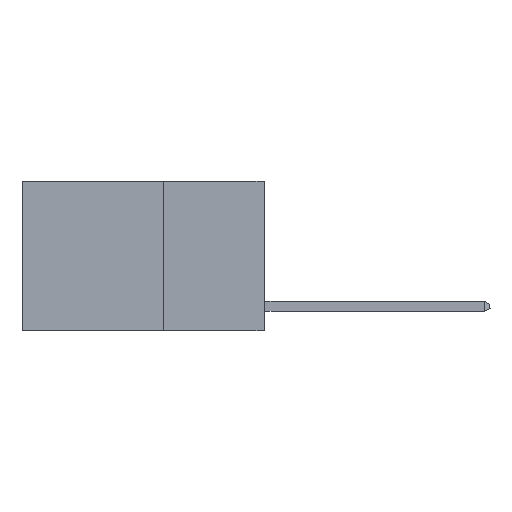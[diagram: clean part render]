
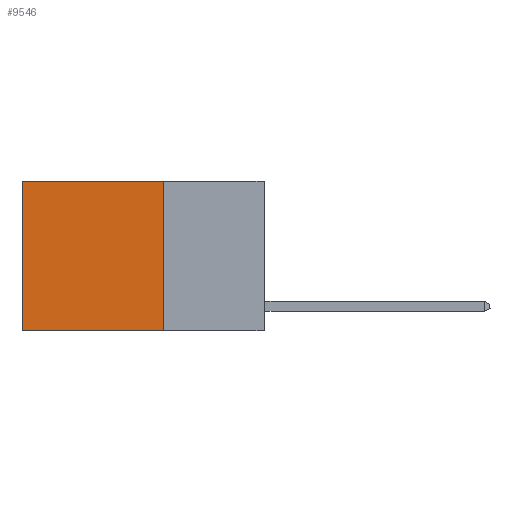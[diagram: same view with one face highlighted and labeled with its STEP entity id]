
A CAD part, left-side view. The second image highlights one B-rep face of the part: STEP entity #9546.
In plain terms, the highlighted planar face has unit normal (-1, 0, 0).
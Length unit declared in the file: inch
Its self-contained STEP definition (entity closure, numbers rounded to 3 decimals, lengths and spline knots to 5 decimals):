
#25 = CARTESIAN_POINT ( 'NONE',  ( 0.2625, 0.6, 0. ) ) ;
#357 = LINE ( 'NONE', #6250, #11164 ) ;
#713 = VERTEX_POINT ( 'NONE', #3164 ) ;
#945 = VERTEX_POINT ( 'NONE', #5092 ) ;
#1223 = ORIENTED_EDGE ( 'NONE', *, *, #12837, .T. ) ;
#1335 = CARTESIAN_POINT ( 'NONE',  ( 0.2625, 0.6, 0. ) ) ;
#2408 = CARTESIAN_POINT ( 'NONE',  ( 0.2625, 0.25, -0.37 ) ) ;
#2613 = VECTOR ( 'NONE', #14532, 39.37008 ) ;
#3164 = CARTESIAN_POINT ( 'NONE',  ( 0.2625, 0.6, -0.37 ) ) ;
#3203 = AXIS2_PLACEMENT_3D ( 'NONE', #6330, #13665, #7483 ) ;
#4871 = DIRECTION ( 'NONE',  ( 0., 1., 0. ) ) ;
#5092 = CARTESIAN_POINT ( 'NONE',  ( 0.2625, 0.25, 0. ) ) ;
#5336 = EDGE_CURVE ( 'NONE', #945, #13176, #8406, .T. ) ;
#5428 = ORIENTED_EDGE ( 'NONE', *, *, #12963, .F. ) ;
#5630 = EDGE_LOOP ( 'NONE', ( #1223, #5428, #9118, #13320 ) ) ;
#6250 = CARTESIAN_POINT ( 'NONE',  ( 0.2625, 0.25, 0. ) ) ;
#6330 = CARTESIAN_POINT ( 'NONE',  ( 0.2625, 0.25, 0. ) ) ;
#7483 = DIRECTION ( 'NONE',  ( 0., 0., -1. ) ) ;
#7679 = LINE ( 'NONE', #7755, #2613 ) ;
#7755 = CARTESIAN_POINT ( 'NONE',  ( 0.2625, 0.25, -0.37 ) ) ;
#8406 = LINE ( 'NONE', #13109, #12519 ) ;
#8458 = DIRECTION ( 'NONE',  ( 0., 0., -1. ) ) ;
#8799 = FACE_OUTER_BOUND ( 'NONE', #5630, .T. ) ;
#9118 = ORIENTED_EDGE ( 'NONE', *, *, #5336, .F. ) ;
#9429 = EDGE_CURVE ( 'NONE', #945, #9751, #357, .T. ) ;
#9546 = ADVANCED_FACE ( 'NONE', ( #8799 ), #14803, .F. ) ;
#9751 = VERTEX_POINT ( 'NONE', #1335 ) ;
#10487 = DIRECTION ( 'NONE',  ( 0., 0., -1. ) ) ;
#11164 = VECTOR ( 'NONE', #4871, 39.37008 ) ;
#12267 = VECTOR ( 'NONE', #8458, 39.37008 ) ;
#12519 = VECTOR ( 'NONE', #10487, 39.37008 ) ;
#12837 = EDGE_CURVE ( 'NONE', #9751, #713, #13166, .T. ) ;
#12963 = EDGE_CURVE ( 'NONE', #13176, #713, #7679, .T. ) ;
#13109 = CARTESIAN_POINT ( 'NONE',  ( 0.2625, 0.25, 0. ) ) ;
#13166 = LINE ( 'NONE', #25, #12267 ) ;
#13176 = VERTEX_POINT ( 'NONE', #2408 ) ;
#13320 = ORIENTED_EDGE ( 'NONE', *, *, #9429, .T. ) ;
#13665 = DIRECTION ( 'NONE',  ( 1., 0., 0. ) ) ;
#14532 = DIRECTION ( 'NONE',  ( 0., 1., 0. ) ) ;
#14803 = PLANE ( 'NONE',  #3203 ) ;
